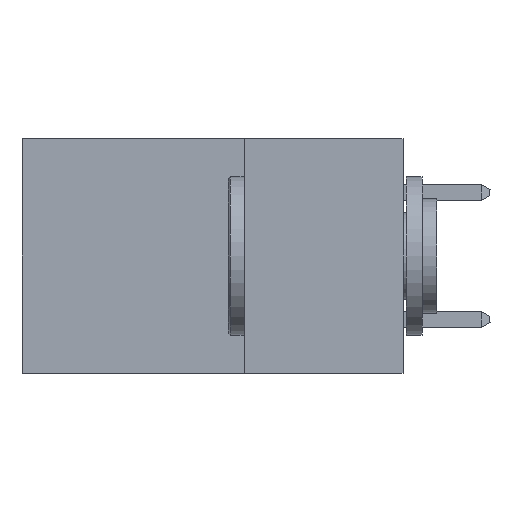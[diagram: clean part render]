
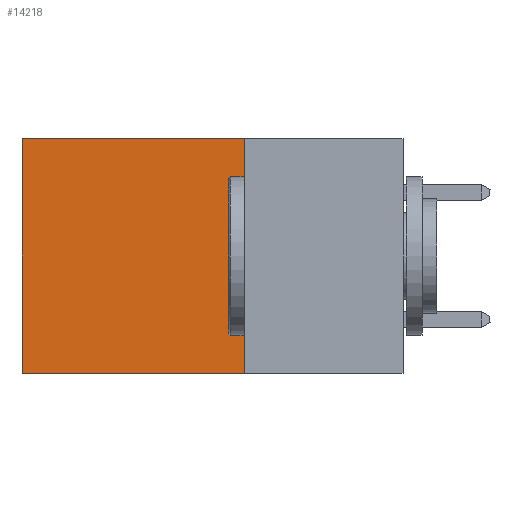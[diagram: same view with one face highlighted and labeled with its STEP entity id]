
A CAD part, left-side view. The second image highlights one B-rep face of the part: STEP entity #14218.
In plain terms, the highlighted planar face has unit normal (-1, 0, 0).
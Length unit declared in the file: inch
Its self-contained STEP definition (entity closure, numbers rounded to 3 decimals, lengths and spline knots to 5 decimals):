
#945 = VECTOR ( 'NONE', #38950, 39.37008 ) ;
#1771 = CARTESIAN_POINT ( 'NONE',  ( 0.2875, 0.25, 0. ) ) ;
#2056 = EDGE_CURVE ( 'NONE', #39875, #21763, #28235, .T. ) ;
#2248 = VECTOR ( 'NONE', #18018, 39.37008 ) ;
#3907 = PLANE ( 'NONE',  #30206 ) ;
#5469 = DIRECTION ( 'NONE',  ( 0., 0., -1. ) ) ;
#8818 = DIRECTION ( 'NONE',  ( 0., 0., -1. ) ) ;
#10351 = FACE_OUTER_BOUND ( 'NONE', #30503, .T. ) ;
#14218 = ADVANCED_FACE ( 'NONE', ( #10351 ), #3907, .F. ) ;
#15815 = CARTESIAN_POINT ( 'NONE',  ( 0.2875, 0.25, -0.37 ) ) ;
#16197 = VECTOR ( 'NONE', #8818, 39.37008 ) ;
#18018 = DIRECTION ( 'NONE',  ( 0., 1., 0. ) ) ;
#18960 = EDGE_CURVE ( 'NONE', #39875, #31703, #42057, .T. ) ;
#19854 = DIRECTION ( 'NONE',  ( 0., 0., -1. ) ) ;
#21606 = ORIENTED_EDGE ( 'NONE', *, *, #36045, .T. ) ;
#21763 = VERTEX_POINT ( 'NONE', #33232 ) ;
#22867 = LINE ( 'NONE', #15815, #945 ) ;
#24706 = CARTESIAN_POINT ( 'NONE',  ( 0.2875, 0.25, 0. ) ) ;
#25079 = CARTESIAN_POINT ( 'NONE',  ( 0.2875, 0.6, -0.37 ) ) ;
#25169 = ORIENTED_EDGE ( 'NONE', *, *, #35035, .F. ) ;
#26320 = VECTOR ( 'NONE', #5469, 39.37008 ) ;
#26713 = DIRECTION ( 'NONE',  ( 1., 0., 0. ) ) ;
#27859 = ORIENTED_EDGE ( 'NONE', *, *, #18960, .F. ) ;
#28235 = LINE ( 'NONE', #24706, #2248 ) ;
#29961 = CARTESIAN_POINT ( 'NONE',  ( 0.2875, 0.25, 0. ) ) ;
#30206 = AXIS2_PLACEMENT_3D ( 'NONE', #29961, #26713, #19854 ) ;
#30503 = EDGE_LOOP ( 'NONE', ( #21606, #25169, #27859, #39116 ) ) ;
#31703 = VERTEX_POINT ( 'NONE', #41716 ) ;
#33232 = CARTESIAN_POINT ( 'NONE',  ( 0.2875, 0.6, 0. ) ) ;
#33630 = VERTEX_POINT ( 'NONE', #25079 ) ;
#35035 = EDGE_CURVE ( 'NONE', #31703, #33630, #22867, .T. ) ;
#35481 = LINE ( 'NONE', #38118, #16197 ) ;
#36045 = EDGE_CURVE ( 'NONE', #21763, #33630, #35481, .T. ) ;
#38118 = CARTESIAN_POINT ( 'NONE',  ( 0.2875, 0.6, 0. ) ) ;
#38950 = DIRECTION ( 'NONE',  ( 0., 1., 0. ) ) ;
#39116 = ORIENTED_EDGE ( 'NONE', *, *, #2056, .T. ) ;
#39875 = VERTEX_POINT ( 'NONE', #40518 ) ;
#40518 = CARTESIAN_POINT ( 'NONE',  ( 0.2875, 0.25, 0. ) ) ;
#41716 = CARTESIAN_POINT ( 'NONE',  ( 0.2875, 0.25, -0.37 ) ) ;
#42057 = LINE ( 'NONE', #1771, #26320 ) ;
